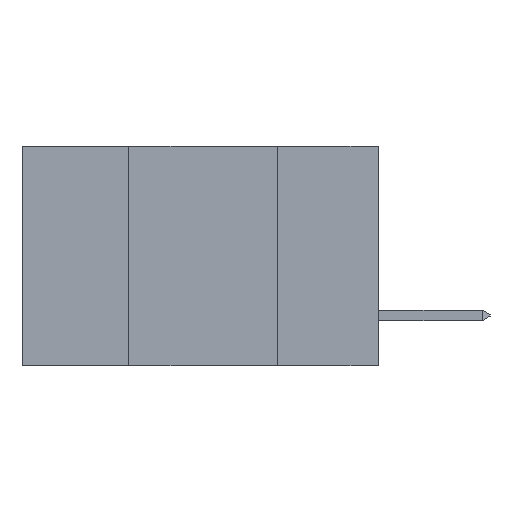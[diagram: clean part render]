
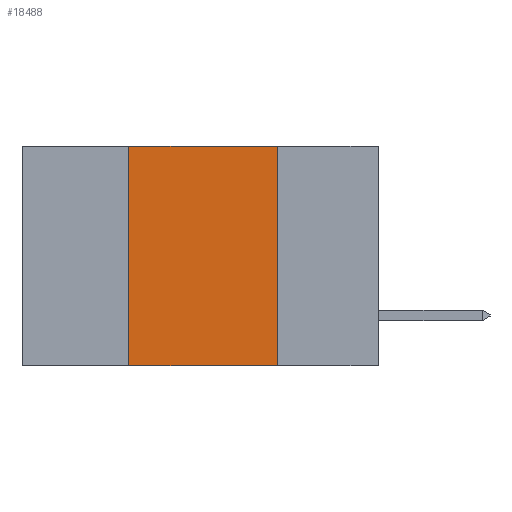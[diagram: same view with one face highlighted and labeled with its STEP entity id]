
A CAD part, left-side view. The second image highlights one B-rep face of the part: STEP entity #18488.
In plain terms, the highlighted planar face has unit normal (-1, 0, 0).
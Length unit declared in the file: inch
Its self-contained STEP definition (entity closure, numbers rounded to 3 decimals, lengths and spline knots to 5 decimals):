
#135 = VECTOR ( 'NONE', #15747, 39.37008 ) ;
#543 = CARTESIAN_POINT ( 'NONE',  ( 0., 0.42, -0.37 ) ) ;
#546 = VERTEX_POINT ( 'NONE', #20995 ) ;
#1007 = ORIENTED_EDGE ( 'NONE', *, *, #9115, .F. ) ;
#1196 = LINE ( 'NONE', #5337, #135 ) ;
#1563 = DIRECTION ( 'NONE',  ( 0., 0., -1. ) ) ;
#1933 = VERTEX_POINT ( 'NONE', #12578 ) ;
#2370 = LINE ( 'NONE', #6634, #7118 ) ;
#3964 = DIRECTION ( 'NONE',  ( 0., -1., 0. ) ) ;
#4626 = VERTEX_POINT ( 'NONE', #543 ) ;
#5337 = CARTESIAN_POINT ( 'NONE',  ( 0., 0.17, -0.37 ) ) ;
#6161 = DIRECTION ( 'NONE',  ( 0., -1., 0. ) ) ;
#6634 = CARTESIAN_POINT ( 'NONE',  ( 0., 0.6, -0.37 ) ) ;
#7118 = VECTOR ( 'NONE', #6161, 39.37008 ) ;
#7359 = LINE ( 'NONE', #9420, #20391 ) ;
#7911 = EDGE_CURVE ( 'NONE', #4626, #8013, #2370, .T. ) ;
#8013 = VERTEX_POINT ( 'NONE', #21283 ) ;
#9115 = EDGE_CURVE ( 'NONE', #4626, #1933, #7359, .T. ) ;
#9306 = CARTESIAN_POINT ( 'NONE',  ( 0., 0.6, 0. ) ) ;
#9420 = CARTESIAN_POINT ( 'NONE',  ( 0., 0.42, -0.37 ) ) ;
#10297 = EDGE_CURVE ( 'NONE', #1933, #546, #13869, .T. ) ;
#11467 = EDGE_CURVE ( 'NONE', #546, #8013, #1196, .T. ) ;
#11896 = EDGE_LOOP ( 'NONE', ( #13671, #12919, #1007, #13177 ) ) ;
#12076 = DIRECTION ( 'NONE',  ( 1., 0., 0. ) ) ;
#12578 = CARTESIAN_POINT ( 'NONE',  ( 0., 0.42, 0. ) ) ;
#12919 = ORIENTED_EDGE ( 'NONE', *, *, #10297, .F. ) ;
#13177 = ORIENTED_EDGE ( 'NONE', *, *, #7911, .T. ) ;
#13671 = ORIENTED_EDGE ( 'NONE', *, *, #11467, .F. ) ;
#13869 = LINE ( 'NONE', #9306, #21554 ) ;
#14073 = AXIS2_PLACEMENT_3D ( 'NONE', #22000, #12076, #1563 ) ;
#15747 = DIRECTION ( 'NONE',  ( 0., 0., -1. ) ) ;
#18488 = ADVANCED_FACE ( 'NONE', ( #19497 ), #18777, .F. ) ;
#18777 = PLANE ( 'NONE',  #14073 ) ;
#19497 = FACE_OUTER_BOUND ( 'NONE', #11896, .T. ) ;
#20391 = VECTOR ( 'NONE', #21185, 39.37008 ) ;
#20995 = CARTESIAN_POINT ( 'NONE',  ( 0., 0.17, 0. ) ) ;
#21185 = DIRECTION ( 'NONE',  ( 0., 0., 1. ) ) ;
#21283 = CARTESIAN_POINT ( 'NONE',  ( 0., 0.17, -0.37 ) ) ;
#21554 = VECTOR ( 'NONE', #3964, 39.37008 ) ;
#22000 = CARTESIAN_POINT ( 'NONE',  ( 0., 0.6, 0. ) ) ;
